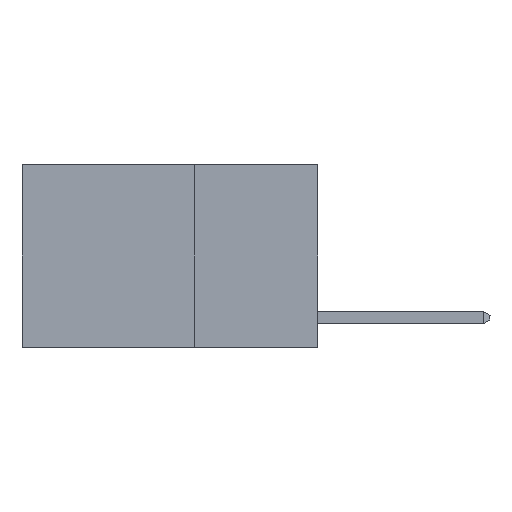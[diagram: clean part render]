
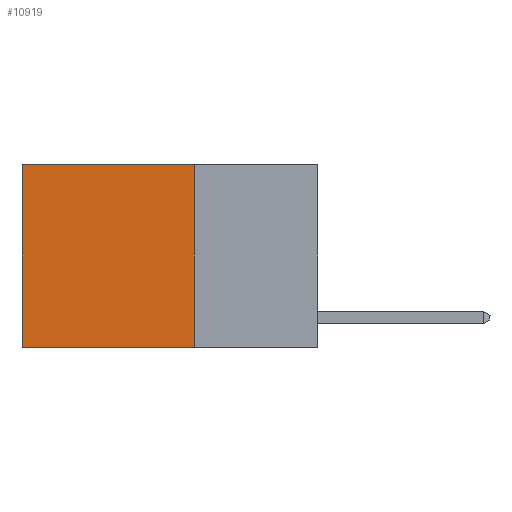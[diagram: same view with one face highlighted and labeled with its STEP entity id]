
A CAD part, left-side view. The second image highlights one B-rep face of the part: STEP entity #10919.
In plain terms, the highlighted planar face has unit normal (-1, 0, 0).
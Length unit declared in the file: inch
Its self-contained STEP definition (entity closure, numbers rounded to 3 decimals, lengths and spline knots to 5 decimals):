
#705 = CARTESIAN_POINT ( 'NONE',  ( 0.2625, 0.6, 0. ) ) ;
#1865 = ORIENTED_EDGE ( 'NONE', *, *, #17067, .T. ) ;
#2063 = LINE ( 'NONE', #17141, #7671 ) ;
#2100 = CARTESIAN_POINT ( 'NONE',  ( 0.2625, 0.25, 0. ) ) ;
#2249 = CARTESIAN_POINT ( 'NONE',  ( 0.2625, 0.6, -0.37 ) ) ;
#4298 = ORIENTED_EDGE ( 'NONE', *, *, #6062, .F. ) ;
#5632 = EDGE_CURVE ( 'NONE', #6352, #20577, #2063, .T. ) ;
#5651 = DIRECTION ( 'NONE',  ( 0., 0., -1. ) ) ;
#5831 = DIRECTION ( 'NONE',  ( 0., 0., -1. ) ) ;
#5903 = DIRECTION ( 'NONE',  ( 1., 0., 0. ) ) ;
#6062 = EDGE_CURVE ( 'NONE', #16036, #20577, #12724, .T. ) ;
#6341 = DIRECTION ( 'NONE',  ( 0., 1., 0. ) ) ;
#6352 = VERTEX_POINT ( 'NONE', #705 ) ;
#7325 = ORIENTED_EDGE ( 'NONE', *, *, #5632, .T. ) ;
#7342 = LINE ( 'NONE', #23174, #16820 ) ;
#7671 = VECTOR ( 'NONE', #5831, 39.37008 ) ;
#9059 = CARTESIAN_POINT ( 'NONE',  ( 0.2625, 0.25, 0. ) ) ;
#9377 = DIRECTION ( 'NONE',  ( 0., 1., 0. ) ) ;
#9458 = CARTESIAN_POINT ( 'NONE',  ( 0.2625, 0.25, 0. ) ) ;
#9788 = ORIENTED_EDGE ( 'NONE', *, *, #10846, .F. ) ;
#10361 = VECTOR ( 'NONE', #5651, 39.37008 ) ;
#10684 = VERTEX_POINT ( 'NONE', #9059 ) ;
#10846 = EDGE_CURVE ( 'NONE', #10684, #16036, #20335, .T. ) ;
#10919 = ADVANCED_FACE ( 'NONE', ( #18583 ), #17202, .F. ) ;
#12137 = VECTOR ( 'NONE', #9377, 39.37008 ) ;
#12724 = LINE ( 'NONE', #20627, #12137 ) ;
#15083 = EDGE_LOOP ( 'NONE', ( #7325, #4298, #9788, #1865 ) ) ;
#16036 = VERTEX_POINT ( 'NONE', #19874 ) ;
#16820 = VECTOR ( 'NONE', #6341, 39.37008 ) ;
#17067 = EDGE_CURVE ( 'NONE', #10684, #6352, #7342, .T. ) ;
#17141 = CARTESIAN_POINT ( 'NONE',  ( 0.2625, 0.6, 0. ) ) ;
#17202 = PLANE ( 'NONE',  #24260 ) ;
#18583 = FACE_OUTER_BOUND ( 'NONE', #15083, .T. ) ;
#19073 = DIRECTION ( 'NONE',  ( 0., 0., -1. ) ) ;
#19874 = CARTESIAN_POINT ( 'NONE',  ( 0.2625, 0.25, -0.37 ) ) ;
#20335 = LINE ( 'NONE', #9458, #10361 ) ;
#20577 = VERTEX_POINT ( 'NONE', #2249 ) ;
#20627 = CARTESIAN_POINT ( 'NONE',  ( 0.2625, 0.25, -0.37 ) ) ;
#23174 = CARTESIAN_POINT ( 'NONE',  ( 0.2625, 0.25, 0. ) ) ;
#24260 = AXIS2_PLACEMENT_3D ( 'NONE', #2100, #5903, #19073 ) ;
